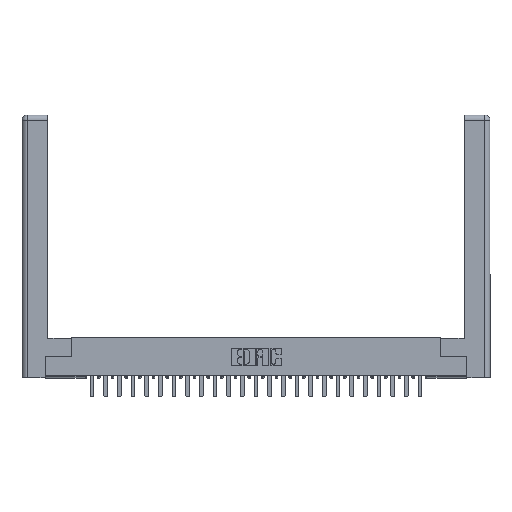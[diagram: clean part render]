
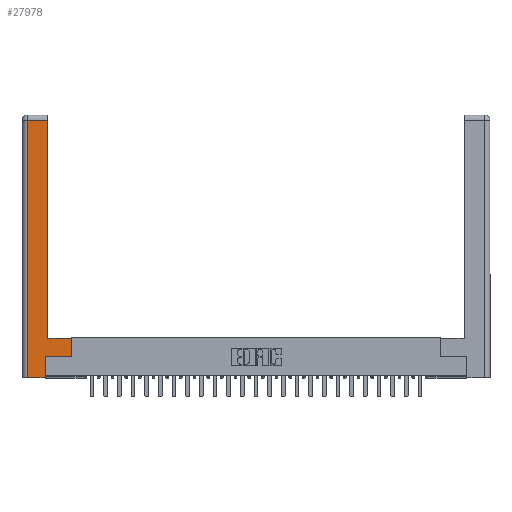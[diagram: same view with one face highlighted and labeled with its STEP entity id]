
A CAD part, top view. The second image highlights one B-rep face of the part: STEP entity #27978.
In plain terms, the highlighted planar face has unit normal (0, 0, 1).
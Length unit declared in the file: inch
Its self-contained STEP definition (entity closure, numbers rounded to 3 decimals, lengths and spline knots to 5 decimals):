
#67 = CARTESIAN_POINT ( 'NONE',  ( 0.265, 0.245, 0. ) ) ;
#767 = ORIENTED_EDGE ( 'NONE', *, *, #2108, .T. ) ;
#788 = CARTESIAN_POINT ( 'NONE',  ( 0.265, 0.245, 0. ) ) ;
#1384 = CARTESIAN_POINT ( 'NONE',  ( 0.565, 0.45, 0. ) ) ;
#1565 = DIRECTION ( 'NONE',  ( 0., 0., -1. ) ) ;
#1990 = FACE_OUTER_BOUND ( 'NONE', #16854, .T. ) ;
#2108 = EDGE_CURVE ( 'NONE', #17903, #3521, #9969, .T. ) ;
#3175 = CARTESIAN_POINT ( 'NONE',  ( 0.565, 0.245, 0. ) ) ;
#3208 = CARTESIAN_POINT ( 'NONE',  ( 0.265, 0., 0. ) ) ;
#3521 = VERTEX_POINT ( 'NONE', #788 ) ;
#4445 = ORIENTED_EDGE ( 'NONE', *, *, #10082, .T. ) ;
#6171 = VERTEX_POINT ( 'NONE', #27748 ) ;
#7309 = VECTOR ( 'NONE', #13213, 39.37008 ) ;
#8273 = VERTEX_POINT ( 'NONE', #20845 ) ;
#8735 = CARTESIAN_POINT ( 'NONE',  ( 0.0615, 2.94, 0. ) ) ;
#8953 = CARTESIAN_POINT ( 'NONE',  ( 0., 0., 0. ) ) ;
#9969 = LINE ( 'NONE', #67, #7309 ) ;
#10082 = EDGE_CURVE ( 'NONE', #27899, #13900, #16899, .T. ) ;
#10256 = DIRECTION ( 'NONE',  ( 1., 0., 0. ) ) ;
#10834 = EDGE_CURVE ( 'NONE', #8273, #6171, #31528, .T. ) ;
#10875 = VERTEX_POINT ( 'NONE', #22619 ) ;
#11156 = ORIENTED_EDGE ( 'NONE', *, *, #11472, .T. ) ;
#11472 = EDGE_CURVE ( 'NONE', #10875, #8273, #23514, .T. ) ;
#11482 = ORIENTED_EDGE ( 'NONE', *, *, #22793, .T. ) ;
#11826 = VECTOR ( 'NONE', #10256, 39.37008 ) ;
#12035 = VECTOR ( 'NONE', #17600, 39.37008 ) ;
#12042 = VECTOR ( 'NONE', #18390, 39.37008 ) ;
#12579 = LINE ( 'NONE', #3175, #11826 ) ;
#13213 = DIRECTION ( 'NONE',  ( 0., 1., 0. ) ) ;
#13900 = VERTEX_POINT ( 'NONE', #18568 ) ;
#14411 = AXIS2_PLACEMENT_3D ( 'NONE', #8953, #1565, #18691 ) ;
#15116 = CARTESIAN_POINT ( 'NONE',  ( 0.295, 0.45, 0. ) ) ;
#15261 = ORIENTED_EDGE ( 'NONE', *, *, #10834, .T. ) ;
#15312 = DIRECTION ( 'NONE',  ( 0., 1., 0. ) ) ;
#15533 = EDGE_CURVE ( 'NONE', #16311, #17903, #16327, .T. ) ;
#15990 = DIRECTION ( 'NONE',  ( -1., 0., 0. ) ) ;
#16311 = VERTEX_POINT ( 'NONE', #26168 ) ;
#16327 = LINE ( 'NONE', #3208, #28536 ) ;
#16751 = LINE ( 'NONE', #30167, #31265 ) ;
#16854 = EDGE_LOOP ( 'NONE', ( #11482, #4445, #18279, #25630, #767, #20171, #11156, #15261 ) ) ;
#16899 = LINE ( 'NONE', #8735, #27568 ) ;
#17600 = DIRECTION ( 'NONE',  ( -1., 0., 0. ) ) ;
#17903 = VERTEX_POINT ( 'NONE', #20213 ) ;
#18004 = DIRECTION ( 'NONE',  ( 0., -1., 0. ) ) ;
#18279 = ORIENTED_EDGE ( 'NONE', *, *, #30319, .T. ) ;
#18390 = DIRECTION ( 'NONE',  ( 0., 1., 0. ) ) ;
#18568 = CARTESIAN_POINT ( 'NONE',  ( 0.0615, 2.94, 0. ) ) ;
#18691 = DIRECTION ( 'NONE',  ( -1., 0., 0. ) ) ;
#18786 = CARTESIAN_POINT ( 'NONE',  ( 0.295, 2.94, 0. ) ) ;
#20171 = ORIENTED_EDGE ( 'NONE', *, *, #22117, .T. ) ;
#20213 = CARTESIAN_POINT ( 'NONE',  ( 0.265, 0., 0. ) ) ;
#20845 = CARTESIAN_POINT ( 'NONE',  ( 0.565, 0.45, 0. ) ) ;
#22117 = EDGE_CURVE ( 'NONE', #3521, #10875, #12579, .T. ) ;
#22619 = CARTESIAN_POINT ( 'NONE',  ( 0.565, 0.245, 0. ) ) ;
#22692 = CARTESIAN_POINT ( 'NONE',  ( 0.0615, 0., 0. ) ) ;
#22793 = EDGE_CURVE ( 'NONE', #6171, #27899, #16751, .T. ) ;
#22973 = VECTOR ( 'NONE', #18004, 39.37008 ) ;
#23514 = LINE ( 'NONE', #1384, #12042 ) ;
#23684 = PLANE ( 'NONE',  #14411 ) ;
#23736 = LINE ( 'NONE', #22692, #22973 ) ;
#25465 = DIRECTION ( 'NONE',  ( 1., 0., 0. ) ) ;
#25630 = ORIENTED_EDGE ( 'NONE', *, *, #15533, .T. ) ;
#26168 = CARTESIAN_POINT ( 'NONE',  ( 0.0615, 0., 0. ) ) ;
#27568 = VECTOR ( 'NONE', #15990, 39.37008 ) ;
#27748 = CARTESIAN_POINT ( 'NONE',  ( 0.295, 0.45, 0. ) ) ;
#27899 = VERTEX_POINT ( 'NONE', #18786 ) ;
#27978 = ADVANCED_FACE ( 'NONE', ( #1990 ), #23684, .F. ) ;
#28536 = VECTOR ( 'NONE', #25465, 39.37008 ) ;
#30167 = CARTESIAN_POINT ( 'NONE',  ( 0.295, 3., 0. ) ) ;
#30319 = EDGE_CURVE ( 'NONE', #13900, #16311, #23736, .T. ) ;
#31265 = VECTOR ( 'NONE', #15312, 39.37008 ) ;
#31528 = LINE ( 'NONE', #15116, #12035 ) ;
